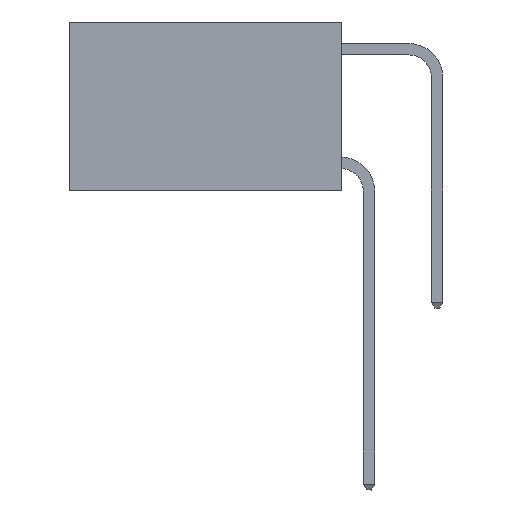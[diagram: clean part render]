
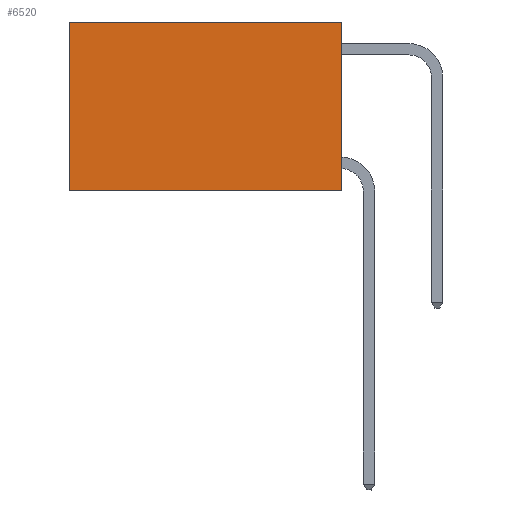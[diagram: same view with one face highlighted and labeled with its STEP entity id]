
A CAD part, left-side view. The second image highlights one B-rep face of the part: STEP entity #6520.
In plain terms, the highlighted planar face has unit normal (-1, 0, 0).
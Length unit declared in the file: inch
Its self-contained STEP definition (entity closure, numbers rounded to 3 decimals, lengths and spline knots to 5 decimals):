
#508 = CARTESIAN_POINT ( 'NONE',  ( 0.2625, 0., -0.37 ) ) ;
#533 = DIRECTION ( 'NONE',  ( 0., 0., -1. ) ) ;
#1028 = EDGE_CURVE ( 'NONE', #11382, #6034, #8449, .T. ) ;
#1081 = ORIENTED_EDGE ( 'NONE', *, *, #10369, .F. ) ;
#1116 = ORIENTED_EDGE ( 'NONE', *, *, #1864, .F. ) ;
#1239 = VECTOR ( 'NONE', #15959, 39.37008 ) ;
#1627 = PLANE ( 'NONE',  #14768 ) ;
#1864 = EDGE_CURVE ( 'NONE', #14261, #9621, #11944, .T. ) ;
#2774 = LINE ( 'NONE', #13175, #15903 ) ;
#2980 = CARTESIAN_POINT ( 'NONE',  ( 0.2625, 0., 0. ) ) ;
#3091 = ORIENTED_EDGE ( 'NONE', *, *, #6276, .T. ) ;
#3161 = CARTESIAN_POINT ( 'NONE',  ( 0.2625, 0., -0.37 ) ) ;
#3434 = VECTOR ( 'NONE', #10005, 39.37008 ) ;
#5973 = CARTESIAN_POINT ( 'NONE',  ( 0.2625, 0.6, -0.37 ) ) ;
#6034 = VERTEX_POINT ( 'NONE', #13311 ) ;
#6276 = EDGE_CURVE ( 'NONE', #6034, #9621, #17288, .T. ) ;
#6495 = VECTOR ( 'NONE', #533, 39.37008 ) ;
#6520 = ADVANCED_FACE ( 'NONE', ( #14109 ), #1627, .F. ) ;
#8449 = LINE ( 'NONE', #10722, #1239 ) ;
#9464 = CARTESIAN_POINT ( 'NONE',  ( 0.2625, 0., 0. ) ) ;
#9621 = VERTEX_POINT ( 'NONE', #5973 ) ;
#10005 = DIRECTION ( 'NONE',  ( 0., 1., 0. ) ) ;
#10233 = DIRECTION ( 'NONE',  ( 0., 0., -1. ) ) ;
#10369 = EDGE_CURVE ( 'NONE', #11382, #14261, #2774, .T. ) ;
#10577 = ORIENTED_EDGE ( 'NONE', *, *, #1028, .T. ) ;
#10722 = CARTESIAN_POINT ( 'NONE',  ( 0.2625, 0., 0. ) ) ;
#11382 = VERTEX_POINT ( 'NONE', #9464 ) ;
#11944 = LINE ( 'NONE', #3161, #3434 ) ;
#12499 = DIRECTION ( 'NONE',  ( 1., 0., 0. ) ) ;
#13175 = CARTESIAN_POINT ( 'NONE',  ( 0.2625, 0., 0. ) ) ;
#13311 = CARTESIAN_POINT ( 'NONE',  ( 0.2625, 0.6, 0. ) ) ;
#13971 = EDGE_LOOP ( 'NONE', ( #3091, #1116, #1081, #10577 ) ) ;
#14109 = FACE_OUTER_BOUND ( 'NONE', #13971, .T. ) ;
#14261 = VERTEX_POINT ( 'NONE', #508 ) ;
#14768 = AXIS2_PLACEMENT_3D ( 'NONE', #2980, #12499, #10233 ) ;
#15346 = CARTESIAN_POINT ( 'NONE',  ( 0.2625, 0.6, 0. ) ) ;
#15903 = VECTOR ( 'NONE', #17422, 39.37008 ) ;
#15959 = DIRECTION ( 'NONE',  ( 0., 1., 0. ) ) ;
#17288 = LINE ( 'NONE', #15346, #6495 ) ;
#17422 = DIRECTION ( 'NONE',  ( 0., 0., -1. ) ) ;
